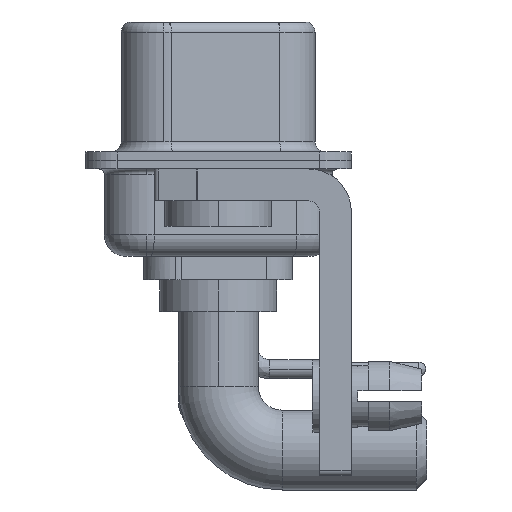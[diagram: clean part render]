
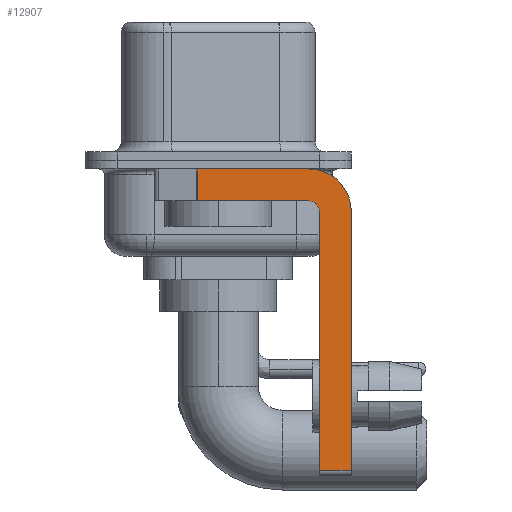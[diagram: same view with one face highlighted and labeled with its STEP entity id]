
A CAD part, left-side view. The second image highlights one B-rep face of the part: STEP entity #12907.
In plain terms, the highlighted planar face has unit normal (-1, 0, 0).
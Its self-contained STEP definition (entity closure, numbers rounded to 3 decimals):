
#580 = VECTOR ( 'NONE', #17984, 1000. ) ;
#1202 = DIRECTION ( 'NONE',  ( 0., 0., -1. ) ) ;
#2471 = EDGE_CURVE ( 'NONE', #9984, #5622, #14902, .T. ) ;
#3144 = LINE ( 'NONE', #17149, #21560 ) ;
#3710 = DIRECTION ( 'NONE',  ( 1., 0., 0. ) ) ;
#4233 = ORIENTED_EDGE ( 'NONE', *, *, #11534, .T. ) ;
#4871 = VERTEX_POINT ( 'NONE', #26080 ) ;
#5141 = CARTESIAN_POINT ( 'NONE',  ( -2.9, 0.978, -1.9 ) ) ;
#5622 = VERTEX_POINT ( 'NONE', #23943 ) ;
#6213 = EDGE_LOOP ( 'NONE', ( #27781, #14112, #18984, #15145, #10142, #4233, #7465, #9832 ) ) ;
#6646 = CARTESIAN_POINT ( 'NONE',  ( -2.9, 3., -0.4 ) ) ;
#6743 = EDGE_CURVE ( 'NONE', #9984, #4871, #25984, .T. ) ;
#6801 = DIRECTION ( 'NONE',  ( 0., -1., 0. ) ) ;
#6999 = CIRCLE ( 'NONE', #21032, 0.5 ) ;
#7357 = EDGE_CURVE ( 'NONE', #23651, #5622, #9729, .T. ) ;
#7465 = ORIENTED_EDGE ( 'NONE', *, *, #12332, .F. ) ;
#8476 = VERTEX_POINT ( 'NONE', #13990 ) ;
#9349 = CARTESIAN_POINT ( 'NONE',  ( -2.9, 0.978, -0.4 ) ) ;
#9729 = LINE ( 'NONE', #28929, #27513 ) ;
#9832 = ORIENTED_EDGE ( 'NONE', *, *, #14292, .F. ) ;
#9916 = DIRECTION ( 'NONE',  ( 0., 0., -1. ) ) ;
#9984 = VERTEX_POINT ( 'NONE', #9349 ) ;
#10142 = ORIENTED_EDGE ( 'NONE', *, *, #24028, .F. ) ;
#11534 = EDGE_CURVE ( 'NONE', #8476, #19295, #15940, .T. ) ;
#12332 = EDGE_CURVE ( 'NONE', #30286, #19295, #29567, .T. ) ;
#12385 = VECTOR ( 'NONE', #6801, 1000. ) ;
#12425 = DIRECTION ( 'NONE',  ( 1., 0., 0. ) ) ;
#12845 = PLANE ( 'NONE',  #29546 ) ;
#12907 = ADVANCED_FACE ( 'NONE', ( #22744 ), #12845, .F. ) ;
#13032 = AXIS2_PLACEMENT_3D ( 'NONE', #27452, #12425, #9916 ) ;
#13871 = EDGE_CURVE ( 'NONE', #28536, #23651, #6999, .T. ) ;
#13990 = CARTESIAN_POINT ( 'NONE',  ( -2.9, -4.75, -14.55 ) ) ;
#14112 = ORIENTED_EDGE ( 'NONE', *, *, #2471, .T. ) ;
#14292 = EDGE_CURVE ( 'NONE', #4871, #30286, #23065, .T. ) ;
#14443 = VECTOR ( 'NONE', #29418, 1000. ) ;
#14736 = DIRECTION ( 'NONE',  ( 0., 0., -1. ) ) ;
#14902 = LINE ( 'NONE', #5141, #29347 ) ;
#15145 = ORIENTED_EDGE ( 'NONE', *, *, #13871, .F. ) ;
#15940 = LINE ( 'NONE', #25222, #580 ) ;
#16981 = CARTESIAN_POINT ( 'NONE',  ( -2.9, -6.25, -2.4 ) ) ;
#17149 = CARTESIAN_POINT ( 'NONE',  ( -2.9, -4.75, -14.8 ) ) ;
#17984 = DIRECTION ( 'NONE',  ( 0., -1., 0. ) ) ;
#18192 = CARTESIAN_POINT ( 'NONE',  ( -2.9, -4.25, -2.4 ) ) ;
#18984 = ORIENTED_EDGE ( 'NONE', *, *, #7357, .F. ) ;
#19295 = VERTEX_POINT ( 'NONE', #22697 ) ;
#20467 = CARTESIAN_POINT ( 'NONE',  ( -2.9, -4.25, -1.9 ) ) ;
#21032 = AXIS2_PLACEMENT_3D ( 'NONE', #18192, #25277, #27795 ) ;
#21560 = VECTOR ( 'NONE', #29271, 1000. ) ;
#22697 = CARTESIAN_POINT ( 'NONE',  ( -2.9, -6.25, -14.55 ) ) ;
#22744 = FACE_OUTER_BOUND ( 'NONE', #6213, .T. ) ;
#23065 = CIRCLE ( 'NONE', #13032, 2. ) ;
#23651 = VERTEX_POINT ( 'NONE', #20467 ) ;
#23943 = CARTESIAN_POINT ( 'NONE',  ( -2.9, 0.978, -1.9 ) ) ;
#24028 = EDGE_CURVE ( 'NONE', #8476, #28536, #3144, .T. ) ;
#24958 = CARTESIAN_POINT ( 'NONE',  ( -2.9, -4.25, -2.4 ) ) ;
#25222 = CARTESIAN_POINT ( 'NONE',  ( -2.9, -4.25, -14.55 ) ) ;
#25277 = DIRECTION ( 'NONE',  ( -1., 0., 0. ) ) ;
#25949 = CARTESIAN_POINT ( 'NONE',  ( -2.9, -4.75, -2.4 ) ) ;
#25984 = LINE ( 'NONE', #6646, #12385 ) ;
#26080 = CARTESIAN_POINT ( 'NONE',  ( -2.9, -4.25, -0.4 ) ) ;
#26717 = DIRECTION ( 'NONE',  ( 0., 1., 0. ) ) ;
#27452 = CARTESIAN_POINT ( 'NONE',  ( -2.9, -4.25, -2.4 ) ) ;
#27513 = VECTOR ( 'NONE', #26717, 1000. ) ;
#27781 = ORIENTED_EDGE ( 'NONE', *, *, #6743, .F. ) ;
#27795 = DIRECTION ( 'NONE',  ( 0., 0., 1. ) ) ;
#27883 = CARTESIAN_POINT ( 'NONE',  ( -2.9, -6.25, -2.4 ) ) ;
#28536 = VERTEX_POINT ( 'NONE', #25949 ) ;
#28929 = CARTESIAN_POINT ( 'NONE',  ( -2.9, -4.25, -1.9 ) ) ;
#29271 = DIRECTION ( 'NONE',  ( 0., 0., 1. ) ) ;
#29347 = VECTOR ( 'NONE', #14736, 1000. ) ;
#29418 = DIRECTION ( 'NONE',  ( 0., 0., -1. ) ) ;
#29546 = AXIS2_PLACEMENT_3D ( 'NONE', #24958, #3710, #1202 ) ;
#29567 = LINE ( 'NONE', #16981, #14443 ) ;
#30286 = VERTEX_POINT ( 'NONE', #27883 ) ;
